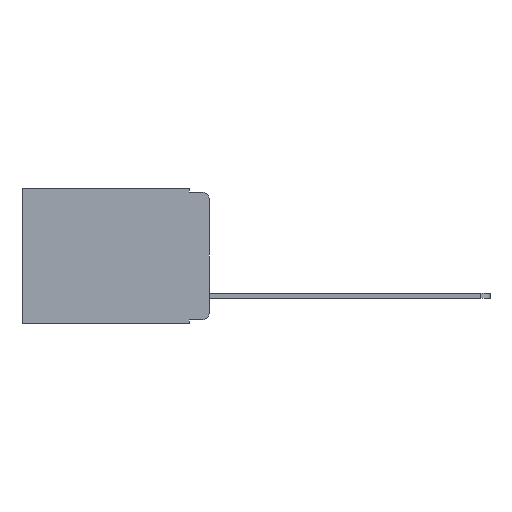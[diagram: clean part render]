
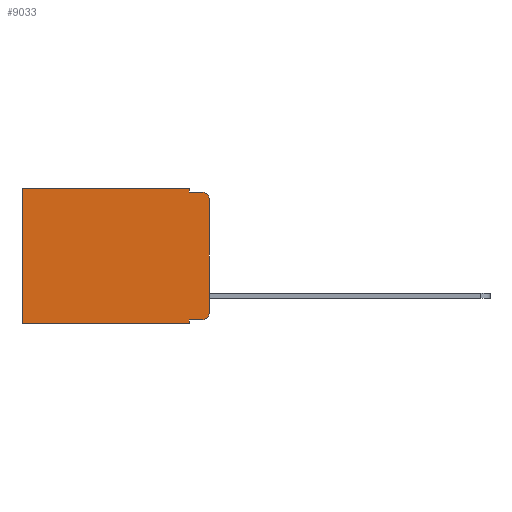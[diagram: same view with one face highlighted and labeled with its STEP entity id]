
A CAD part, left-side view. The second image highlights one B-rep face of the part: STEP entity #9033.
In plain terms, the highlighted planar face has unit normal (-1, 0, 0).
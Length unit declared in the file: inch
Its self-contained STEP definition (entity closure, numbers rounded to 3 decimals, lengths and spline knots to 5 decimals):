
#281 = DIRECTION ( 'NONE',  ( 0., 1., 0. ) ) ;
#386 = CARTESIAN_POINT ( 'NONE',  ( 0.298, 0., 0. ) ) ;
#448 = LINE ( 'NONE', #11139, #9982 ) ;
#537 = DIRECTION ( 'NONE',  ( 1., 0., 0. ) ) ;
#571 = VECTOR ( 'NONE', #11278, 39.37008 ) ;
#724 = EDGE_CURVE ( 'NONE', #2824, #3469, #5927, .T. ) ;
#877 = EDGE_LOOP ( 'NONE', ( #8906, #10389, #9506, #10347, #10232, #10173, #10145, #10048, #10043, #9905 ) ) ;
#897 = VERTEX_POINT ( 'NONE', #1239 ) ;
#918 = AXIS2_PLACEMENT_3D ( 'NONE', #6650, #537, #7554 ) ;
#1098 = EDGE_CURVE ( 'NONE', #10923, #897, #448, .T. ) ;
#1239 = CARTESIAN_POINT ( 'NONE',  ( 0.298, 0.051, -0.343 ) ) ;
#1487 = DIRECTION ( 'NONE',  ( 0., 1., 0. ) ) ;
#1556 = AXIS2_PLACEMENT_3D ( 'NONE', #11841, #5154, #5183 ) ;
#2159 = VECTOR ( 'NONE', #6882, 39.37008 ) ;
#2185 = EDGE_CURVE ( 'NONE', #897, #2576, #4545, .T. ) ;
#2460 = EDGE_CURVE ( 'NONE', #7425, #2576, #11994, .T. ) ;
#2493 = EDGE_CURVE ( 'NONE', #2824, #8982, #7368, .T. ) ;
#2576 = VERTEX_POINT ( 'NONE', #9239 ) ;
#2607 = EDGE_CURVE ( 'NONE', #6560, #8982, #9688, .T. ) ;
#2624 = EDGE_CURVE ( 'NONE', #8495, #6560, #7480, .T. ) ;
#2686 = EDGE_CURVE ( 'NONE', #11337, #3469, #6325, .T. ) ;
#2705 = EDGE_CURVE ( 'NONE', #10923, #11337, #4068, .T. ) ;
#2824 = VERTEX_POINT ( 'NONE', #6431 ) ;
#3377 = VECTOR ( 'NONE', #5776, 39.37008 ) ;
#3469 = VERTEX_POINT ( 'NONE', #9686 ) ;
#3767 = DIRECTION ( 'NONE',  ( 0., 0., -1. ) ) ;
#4018 = DIRECTION ( 'NONE',  ( 0., 0., -1. ) ) ;
#4068 = LINE ( 'NONE', #7538, #571 ) ;
#4109 = CARTESIAN_POINT ( 'NONE',  ( 0.298, 0.473, 0. ) ) ;
#4145 = CARTESIAN_POINT ( 'NONE',  ( 0.298, 0., 0. ) ) ;
#4295 = LINE ( 'NONE', #386, #6561 ) ;
#4545 = LINE ( 'NONE', #4749, #8541 ) ;
#4635 = CARTESIAN_POINT ( 'NONE',  ( 0.298, 0.02, -0.313 ) ) ;
#4686 = VECTOR ( 'NONE', #3767, 39.37008 ) ;
#4695 = CARTESIAN_POINT ( 'NONE',  ( 0.298, 0.051, 0. ) ) ;
#4749 = CARTESIAN_POINT ( 'NONE',  ( 0.298, 0., -0.343 ) ) ;
#4973 = VECTOR ( 'NONE', #5831, 39.37008 ) ;
#5010 = FACE_OUTER_BOUND ( 'NONE', #877, .T. ) ;
#5154 = DIRECTION ( 'NONE',  ( -1., 0., 0. ) ) ;
#5183 = DIRECTION ( 'NONE',  ( 0., 0., -1. ) ) ;
#5223 = CARTESIAN_POINT ( 'NONE',  ( 0.298, 0.051, -0.01 ) ) ;
#5666 = CARTESIAN_POINT ( 'NONE',  ( 0.298, 0.473, 0. ) ) ;
#5776 = DIRECTION ( 'NONE',  ( 0., 0., -1. ) ) ;
#5831 = DIRECTION ( 'NONE',  ( 0., -1., 0. ) ) ;
#5927 = LINE ( 'NONE', #4145, #3377 ) ;
#6325 = CIRCLE ( 'NONE', #10248, 0.02 ) ;
#6431 = CARTESIAN_POINT ( 'NONE',  ( 0.298, 0., -0.03 ) ) ;
#6560 = VERTEX_POINT ( 'NONE', #9308 ) ;
#6561 = VECTOR ( 'NONE', #281, 39.37008 ) ;
#6650 = CARTESIAN_POINT ( 'NONE',  ( 0.298, 0., 0. ) ) ;
#6882 = DIRECTION ( 'NONE',  ( 0., 0., -1. ) ) ;
#6984 = DIRECTION ( 'NONE',  ( -1., 0., 0. ) ) ;
#6992 = EDGE_CURVE ( 'NONE', #8495, #7425, #4295, .T. ) ;
#7368 = CIRCLE ( 'NONE', #1556, 0.02 ) ;
#7425 = VERTEX_POINT ( 'NONE', #4109 ) ;
#7480 = LINE ( 'NONE', #10238, #4686 ) ;
#7538 = CARTESIAN_POINT ( 'NONE',  ( 0.298, 0.051, -0.333 ) ) ;
#7554 = DIRECTION ( 'NONE',  ( 0., 0., -1. ) ) ;
#8495 = VERTEX_POINT ( 'NONE', #4695 ) ;
#8541 = VECTOR ( 'NONE', #1487, 39.37008 ) ;
#8881 = CARTESIAN_POINT ( 'NONE',  ( 0.298, 0.02, -0.333 ) ) ;
#8906 = ORIENTED_EDGE ( 'NONE', *, *, #724, .F. ) ;
#8982 = VERTEX_POINT ( 'NONE', #9077 ) ;
#9033 = ADVANCED_FACE ( 'NONE', ( #5010 ), #9194, .F. ) ;
#9077 = CARTESIAN_POINT ( 'NONE',  ( 0.298, 0.02, -0.01 ) ) ;
#9194 = PLANE ( 'NONE',  #918 ) ;
#9239 = CARTESIAN_POINT ( 'NONE',  ( 0.298, 0.473, -0.343 ) ) ;
#9308 = CARTESIAN_POINT ( 'NONE',  ( 0.298, 0.051, -0.01 ) ) ;
#9506 = ORIENTED_EDGE ( 'NONE', *, *, #2607, .F. ) ;
#9686 = CARTESIAN_POINT ( 'NONE',  ( 0.298, 0., -0.313 ) ) ;
#9688 = LINE ( 'NONE', #5223, #4973 ) ;
#9905 = ORIENTED_EDGE ( 'NONE', *, *, #2686, .T. ) ;
#9982 = VECTOR ( 'NONE', #10448, 39.37008 ) ;
#10043 = ORIENTED_EDGE ( 'NONE', *, *, #2705, .T. ) ;
#10048 = ORIENTED_EDGE ( 'NONE', *, *, #1098, .F. ) ;
#10145 = ORIENTED_EDGE ( 'NONE', *, *, #2185, .F. ) ;
#10173 = ORIENTED_EDGE ( 'NONE', *, *, #2460, .T. ) ;
#10232 = ORIENTED_EDGE ( 'NONE', *, *, #6992, .T. ) ;
#10238 = CARTESIAN_POINT ( 'NONE',  ( 0.298, 0.051, 0. ) ) ;
#10248 = AXIS2_PLACEMENT_3D ( 'NONE', #4635, #6984, #4018 ) ;
#10347 = ORIENTED_EDGE ( 'NONE', *, *, #2624, .F. ) ;
#10389 = ORIENTED_EDGE ( 'NONE', *, *, #2493, .T. ) ;
#10448 = DIRECTION ( 'NONE',  ( 0., 0., -1. ) ) ;
#10923 = VERTEX_POINT ( 'NONE', #11675 ) ;
#11139 = CARTESIAN_POINT ( 'NONE',  ( 0.298, 0.051, 0. ) ) ;
#11278 = DIRECTION ( 'NONE',  ( 0., -1., 0. ) ) ;
#11337 = VERTEX_POINT ( 'NONE', #8881 ) ;
#11675 = CARTESIAN_POINT ( 'NONE',  ( 0.298, 0.051, -0.333 ) ) ;
#11841 = CARTESIAN_POINT ( 'NONE',  ( 0.298, 0.02, -0.03 ) ) ;
#11994 = LINE ( 'NONE', #5666, #2159 ) ;
